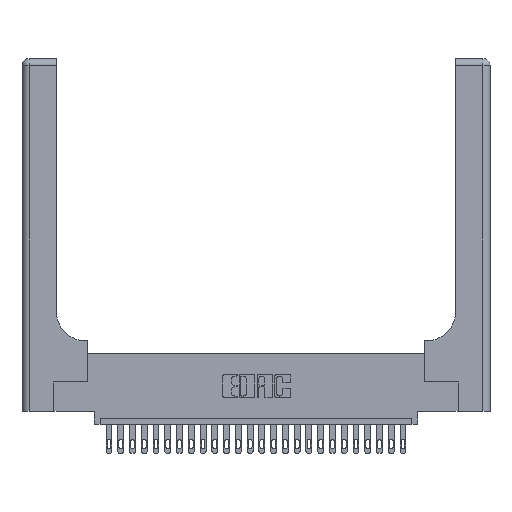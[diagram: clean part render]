
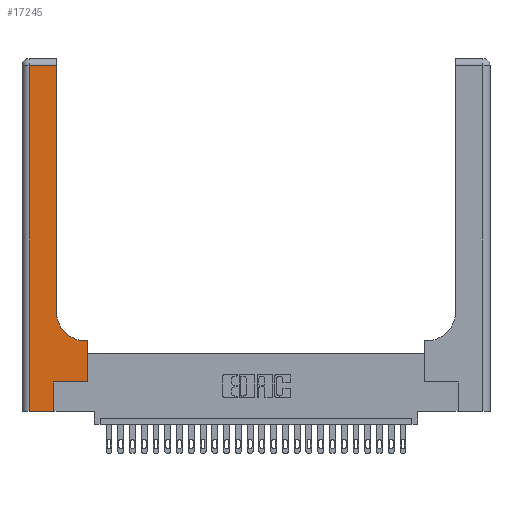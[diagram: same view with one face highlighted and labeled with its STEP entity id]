
A CAD part, top view. The second image highlights one B-rep face of the part: STEP entity #17245.
In plain terms, the highlighted planar face has unit normal (0, 0, 1).
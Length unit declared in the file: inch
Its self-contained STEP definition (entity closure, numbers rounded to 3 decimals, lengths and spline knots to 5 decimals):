
#391 = CARTESIAN_POINT ( 'NONE',  ( 0.269, 0.25, 0.37 ) ) ;
#896 = AXIS2_PLACEMENT_3D ( 'NONE', #12226, #16394, #5856 ) ;
#1536 = CIRCLE ( 'NONE', #7352, 0.25 ) ;
#1710 = LINE ( 'NONE', #7761, #22576 ) ;
#1864 = ORIENTED_EDGE ( 'NONE', *, *, #12374, .T. ) ;
#2118 = LINE ( 'NONE', #3097, #3748 ) ;
#2550 = CARTESIAN_POINT ( 'NONE',  ( 0.06, 3., 0.37 ) ) ;
#2945 = VECTOR ( 'NONE', #12362, 39.37008 ) ;
#3003 = DIRECTION ( 'NONE',  ( 0., 1., 0. ) ) ;
#3097 = CARTESIAN_POINT ( 'NONE',  ( 0.5585, 0.25, 0.37 ) ) ;
#3402 = VERTEX_POINT ( 'NONE', #25671 ) ;
#3748 = VECTOR ( 'NONE', #3003, 39.37008 ) ;
#3882 = ORIENTED_EDGE ( 'NONE', *, *, #4522, .T. ) ;
#4522 = EDGE_CURVE ( 'NONE', #13619, #24037, #8509, .T. ) ;
#5073 = CARTESIAN_POINT ( 'NONE',  ( 0.06, 0., 0.37 ) ) ;
#5705 = CARTESIAN_POINT ( 'NONE',  ( 0., 0., 0.37 ) ) ;
#5856 = DIRECTION ( 'NONE',  ( -1., 0., 0. ) ) ;
#6170 = EDGE_CURVE ( 'NONE', #19537, #18337, #16201, .T. ) ;
#6795 = EDGE_LOOP ( 'NONE', ( #15210, #18384, #22009, #15651, #1864, #19382, #17426, #3882, #8545 ) ) ;
#6983 = CARTESIAN_POINT ( 'NONE',  ( 0.2915, 2.94, 0.37 ) ) ;
#7150 = VERTEX_POINT ( 'NONE', #391 ) ;
#7352 = AXIS2_PLACEMENT_3D ( 'NONE', #19988, #24062, #26414 ) ;
#7761 = CARTESIAN_POINT ( 'NONE',  ( 0.2915, 3., 0.37 ) ) ;
#8036 = PLANE ( 'NONE',  #896 ) ;
#8143 = EDGE_CURVE ( 'NONE', #18337, #3402, #20417, .T. ) ;
#8362 = CARTESIAN_POINT ( 'NONE',  ( 0.2915, 0.6, 0.37 ) ) ;
#8509 = LINE ( 'NONE', #8362, #2945 ) ;
#8545 = ORIENTED_EDGE ( 'NONE', *, *, #15609, .T. ) ;
#8944 = DIRECTION ( 'NONE',  ( 0., -1., 0. ) ) ;
#9138 = CARTESIAN_POINT ( 'NONE',  ( 0.5585, 0.6, 0.37 ) ) ;
#9721 = EDGE_CURVE ( 'NONE', #23564, #19537, #13562, .T. ) ;
#9816 = DIRECTION ( 'NONE',  ( 1., 0., 0. ) ) ;
#9944 = CARTESIAN_POINT ( 'NONE',  ( 0.269, 0., 0.37 ) ) ;
#11899 = VERTEX_POINT ( 'NONE', #17136 ) ;
#12226 = CARTESIAN_POINT ( 'NONE',  ( 0., 3., 0.37 ) ) ;
#12362 = DIRECTION ( 'NONE',  ( -1., 0., 0. ) ) ;
#12374 = EDGE_CURVE ( 'NONE', #3402, #7150, #16288, .T. ) ;
#13562 = LINE ( 'NONE', #22816, #23934 ) ;
#13619 = VERTEX_POINT ( 'NONE', #9138 ) ;
#13773 = DIRECTION ( 'NONE',  ( 0., 1., 0. ) ) ;
#14064 = VECTOR ( 'NONE', #9816, 39.37008 ) ;
#14570 = VERTEX_POINT ( 'NONE', #24728 ) ;
#15210 = ORIENTED_EDGE ( 'NONE', *, *, #22457, .T. ) ;
#15385 = LINE ( 'NONE', #18340, #14064 ) ;
#15609 = EDGE_CURVE ( 'NONE', #24037, #11899, #1536, .T. ) ;
#15651 = ORIENTED_EDGE ( 'NONE', *, *, #8143, .T. ) ;
#16201 = LINE ( 'NONE', #2550, #19479 ) ;
#16288 = LINE ( 'NONE', #9944, #21203 ) ;
#16394 = DIRECTION ( 'NONE',  ( 0., 0., -1. ) ) ;
#16639 = DIRECTION ( 'NONE',  ( -1., 0., 0. ) ) ;
#17136 = CARTESIAN_POINT ( 'NONE',  ( 0.2915, 0.85, 0.37 ) ) ;
#17143 = CARTESIAN_POINT ( 'NONE',  ( 0.5415, 0.6, 0.37 ) ) ;
#17245 = ADVANCED_FACE ( 'NONE', ( #23325 ), #8036, .F. ) ;
#17426 = ORIENTED_EDGE ( 'NONE', *, *, #17707, .T. ) ;
#17670 = CARTESIAN_POINT ( 'NONE',  ( 0.06, 2.94, 0.37 ) ) ;
#17707 = EDGE_CURVE ( 'NONE', #14570, #13619, #2118, .T. ) ;
#18337 = VERTEX_POINT ( 'NONE', #5073 ) ;
#18340 = CARTESIAN_POINT ( 'NONE',  ( 0.269, 0.25, 0.37 ) ) ;
#18384 = ORIENTED_EDGE ( 'NONE', *, *, #9721, .T. ) ;
#19382 = ORIENTED_EDGE ( 'NONE', *, *, #23205, .T. ) ;
#19479 = VECTOR ( 'NONE', #8944, 39.37008 ) ;
#19537 = VERTEX_POINT ( 'NONE', #17670 ) ;
#19988 = CARTESIAN_POINT ( 'NONE',  ( 0.5415, 0.85, 0.37 ) ) ;
#20417 = LINE ( 'NONE', #5705, #23022 ) ;
#21203 = VECTOR ( 'NONE', #26550, 39.37008 ) ;
#22009 = ORIENTED_EDGE ( 'NONE', *, *, #6170, .T. ) ;
#22457 = EDGE_CURVE ( 'NONE', #11899, #23564, #1710, .T. ) ;
#22576 = VECTOR ( 'NONE', #13773, 39.37008 ) ;
#22816 = CARTESIAN_POINT ( 'NONE',  ( 0., 2.94, 0.37 ) ) ;
#23022 = VECTOR ( 'NONE', #26080, 39.37008 ) ;
#23205 = EDGE_CURVE ( 'NONE', #7150, #14570, #15385, .T. ) ;
#23325 = FACE_OUTER_BOUND ( 'NONE', #6795, .T. ) ;
#23564 = VERTEX_POINT ( 'NONE', #6983 ) ;
#23934 = VECTOR ( 'NONE', #16639, 39.37008 ) ;
#24037 = VERTEX_POINT ( 'NONE', #17143 ) ;
#24062 = DIRECTION ( 'NONE',  ( 0., 0., -1. ) ) ;
#24728 = CARTESIAN_POINT ( 'NONE',  ( 0.5585, 0.25, 0.37 ) ) ;
#25671 = CARTESIAN_POINT ( 'NONE',  ( 0.269, 0., 0.37 ) ) ;
#26080 = DIRECTION ( 'NONE',  ( 1., 0., 0. ) ) ;
#26414 = DIRECTION ( 'NONE',  ( 1., 0., 0. ) ) ;
#26550 = DIRECTION ( 'NONE',  ( 0., 1., 0. ) ) ;
